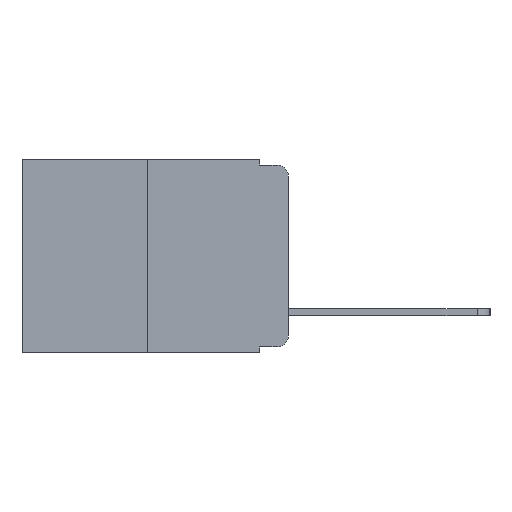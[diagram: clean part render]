
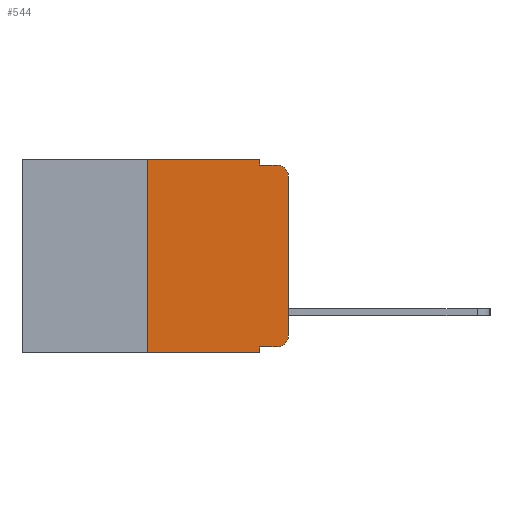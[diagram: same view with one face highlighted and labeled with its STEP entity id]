
A CAD part, left-side view. The second image highlights one B-rep face of the part: STEP entity #544.
In plain terms, the highlighted planar face has unit normal (-1, 0, 0).
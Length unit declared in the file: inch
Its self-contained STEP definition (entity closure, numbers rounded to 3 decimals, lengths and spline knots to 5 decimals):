
#240 = VERTEX_POINT ( 'NONE', #12050 ) ;
#336 = VERTEX_POINT ( 'NONE', #4977 ) ;
#544 = ADVANCED_FACE ( 'NONE', ( #13728 ), #3781, .F. ) ;
#549 = VECTOR ( 'NONE', #1776, 39.37008 ) ;
#736 = DIRECTION ( 'NONE',  ( 0., 0., -1. ) ) ;
#814 = VERTEX_POINT ( 'NONE', #12363 ) ;
#904 = ORIENTED_EDGE ( 'NONE', *, *, #7699, .F. ) ;
#937 = VERTEX_POINT ( 'NONE', #13042 ) ;
#953 = VERTEX_POINT ( 'NONE', #9500 ) ;
#1632 = DIRECTION ( 'NONE',  ( 1., 0., 0. ) ) ;
#1655 = CARTESIAN_POINT ( 'NONE',  ( 0., 0.473, 0. ) ) ;
#1675 = DIRECTION ( 'NONE',  ( -1., 0., 0. ) ) ;
#1776 = DIRECTION ( 'NONE',  ( 0., -1., 0. ) ) ;
#1851 = VECTOR ( 'NONE', #11350, 39.37008 ) ;
#1873 = EDGE_CURVE ( 'NONE', #336, #9133, #12283, .T. ) ;
#2498 = DIRECTION ( 'NONE',  ( 0., 0., -1. ) ) ;
#2761 = CARTESIAN_POINT ( 'NONE',  ( 0., 0.051, -0.333 ) ) ;
#2830 = CARTESIAN_POINT ( 'NONE',  ( 0., 0., 0. ) ) ;
#3089 = CARTESIAN_POINT ( 'NONE',  ( 0., 0., -0.03 ) ) ;
#3119 = LINE ( 'NONE', #2830, #11434 ) ;
#3173 = CARTESIAN_POINT ( 'NONE',  ( 0., 0.25, 0. ) ) ;
#3276 = VECTOR ( 'NONE', #13431, 39.37008 ) ;
#3723 = AXIS2_PLACEMENT_3D ( 'NONE', #8401, #1675, #9482 ) ;
#3781 = PLANE ( 'NONE',  #9939 ) ;
#3791 = CARTESIAN_POINT ( 'NONE',  ( 0., 0.051, -0.333 ) ) ;
#4293 = ORIENTED_EDGE ( 'NONE', *, *, #5130, .F. ) ;
#4723 = EDGE_CURVE ( 'NONE', #8780, #937, #11427, .T. ) ;
#4840 = EDGE_CURVE ( 'NONE', #9133, #814, #11909, .T. ) ;
#4956 = ORIENTED_EDGE ( 'NONE', *, *, #8863, .T. ) ;
#4977 = CARTESIAN_POINT ( 'NONE',  ( 0., 0.25, 0. ) ) ;
#5024 = VECTOR ( 'NONE', #2498, 39.37008 ) ;
#5043 = EDGE_CURVE ( 'NONE', #953, #937, #9626, .T. ) ;
#5116 = CARTESIAN_POINT ( 'NONE',  ( 0., 0., -0.313 ) ) ;
#5130 = EDGE_CURVE ( 'NONE', #814, #240, #5723, .T. ) ;
#5154 = ORIENTED_EDGE ( 'NONE', *, *, #5043, .T. ) ;
#5494 = ORIENTED_EDGE ( 'NONE', *, *, #4723, .F. ) ;
#5723 = LINE ( 'NONE', #7773, #11093 ) ;
#5839 = CARTESIAN_POINT ( 'NONE',  ( 0., 0.051, 0. ) ) ;
#5979 = VECTOR ( 'NONE', #8955, 39.37008 ) ;
#6182 = ORIENTED_EDGE ( 'NONE', *, *, #1873, .F. ) ;
#6246 = VERTEX_POINT ( 'NONE', #3089 ) ;
#7305 = DIRECTION ( 'NONE',  ( 0., 0., 1. ) ) ;
#7437 = CARTESIAN_POINT ( 'NONE',  ( 0., 0.473, -0.343 ) ) ;
#7652 = DIRECTION ( 'NONE',  ( -1., 0., 0. ) ) ;
#7699 = EDGE_CURVE ( 'NONE', #953, #336, #11693, .T. ) ;
#7749 = CARTESIAN_POINT ( 'NONE',  ( 0., 0.051, 0. ) ) ;
#7773 = CARTESIAN_POINT ( 'NONE',  ( 0., 0.051, -0.01 ) ) ;
#7833 = AXIS2_PLACEMENT_3D ( 'NONE', #13838, #7652, #736 ) ;
#8026 = ORIENTED_EDGE ( 'NONE', *, *, #12232, .T. ) ;
#8401 = CARTESIAN_POINT ( 'NONE',  ( 0., 0.02, -0.03 ) ) ;
#8780 = VERTEX_POINT ( 'NONE', #2761 ) ;
#8863 = EDGE_CURVE ( 'NONE', #6246, #240, #12302, .T. ) ;
#8917 = VECTOR ( 'NONE', #10794, 39.37008 ) ;
#8955 = DIRECTION ( 'NONE',  ( 0., -1., 0. ) ) ;
#9133 = VERTEX_POINT ( 'NONE', #7749 ) ;
#9412 = ORIENTED_EDGE ( 'NONE', *, *, #10702, .T. ) ;
#9482 = DIRECTION ( 'NONE',  ( 0., 0., -1. ) ) ;
#9500 = CARTESIAN_POINT ( 'NONE',  ( 0., 0.25, -0.343 ) ) ;
#9626 = LINE ( 'NONE', #7437, #549 ) ;
#9770 = CARTESIAN_POINT ( 'NONE',  ( 0., 0.473, 0. ) ) ;
#9931 = VERTEX_POINT ( 'NONE', #10094 ) ;
#9939 = AXIS2_PLACEMENT_3D ( 'NONE', #1655, #1632, #11099 ) ;
#10094 = CARTESIAN_POINT ( 'NONE',  ( 0., 0.02, -0.333 ) ) ;
#10673 = LINE ( 'NONE', #3791, #1851 ) ;
#10702 = EDGE_CURVE ( 'NONE', #8780, #9931, #10673, .T. ) ;
#10747 = ORIENTED_EDGE ( 'NONE', *, *, #4840, .F. ) ;
#10794 = DIRECTION ( 'NONE',  ( 0., 0., 1. ) ) ;
#11093 = VECTOR ( 'NONE', #12950, 39.37008 ) ;
#11099 = DIRECTION ( 'NONE',  ( 0., 0., -1. ) ) ;
#11350 = DIRECTION ( 'NONE',  ( 0., -1., 0. ) ) ;
#11401 = CARTESIAN_POINT ( 'NONE',  ( 0., 0.051, 0. ) ) ;
#11427 = LINE ( 'NONE', #5839, #5024 ) ;
#11434 = VECTOR ( 'NONE', #7305, 39.37008 ) ;
#11693 = LINE ( 'NONE', #3173, #8917 ) ;
#11909 = LINE ( 'NONE', #11401, #3276 ) ;
#12050 = CARTESIAN_POINT ( 'NONE',  ( 0., 0.02, -0.01 ) ) ;
#12232 = EDGE_CURVE ( 'NONE', #13520, #6246, #3119, .T. ) ;
#12283 = LINE ( 'NONE', #9770, #5979 ) ;
#12302 = CIRCLE ( 'NONE', #3723, 0.02 ) ;
#12363 = CARTESIAN_POINT ( 'NONE',  ( 0., 0.051, -0.01 ) ) ;
#12487 = ORIENTED_EDGE ( 'NONE', *, *, #13032, .T. ) ;
#12950 = DIRECTION ( 'NONE',  ( 0., -1., 0. ) ) ;
#13032 = EDGE_CURVE ( 'NONE', #9931, #13520, #13802, .T. ) ;
#13042 = CARTESIAN_POINT ( 'NONE',  ( 0., 0.051, -0.343 ) ) ;
#13431 = DIRECTION ( 'NONE',  ( 0., 0., -1. ) ) ;
#13433 = EDGE_LOOP ( 'NONE', ( #8026, #4956, #4293, #10747, #6182, #904, #5154, #5494, #9412, #12487 ) ) ;
#13520 = VERTEX_POINT ( 'NONE', #5116 ) ;
#13728 = FACE_OUTER_BOUND ( 'NONE', #13433, .T. ) ;
#13802 = CIRCLE ( 'NONE', #7833, 0.02 ) ;
#13838 = CARTESIAN_POINT ( 'NONE',  ( 0., 0.02, -0.313 ) ) ;
